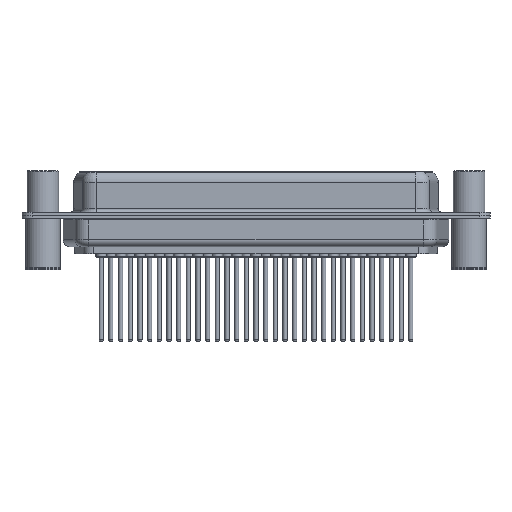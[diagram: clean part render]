
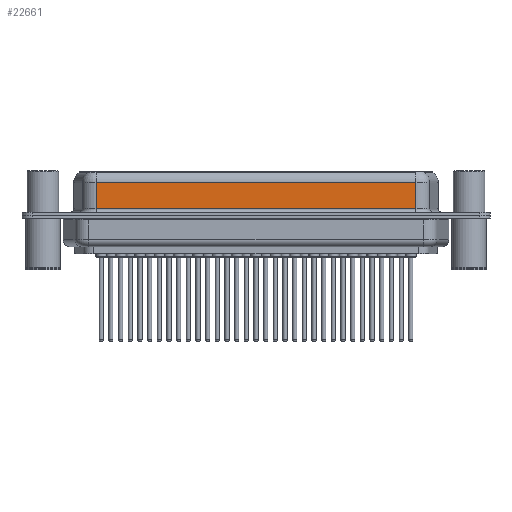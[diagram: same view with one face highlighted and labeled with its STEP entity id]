
A CAD part, front view. The second image highlights one B-rep face of the part: STEP entity #22661.
In plain terms, the highlighted planar face has unit normal (0, -1, 0).
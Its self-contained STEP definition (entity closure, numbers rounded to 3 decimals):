
#1103 = EDGE_CURVE ( 'NONE', #14342, #23252, #28003, .T. ) ;
#1141 = DIRECTION ( 'NONE',  ( 0., 0., -1. ) ) ;
#2949 = EDGE_CURVE ( 'NONE', #29314, #4065, #27001, .T. ) ;
#4065 = VERTEX_POINT ( 'NONE', #7651 ) ;
#4197 = VECTOR ( 'NONE', #24538, 1000. ) ;
#5983 = CARTESIAN_POINT ( 'NONE',  ( 53.383, -5.45, 4.65 ) ) ;
#6524 = LINE ( 'NONE', #5983, #13009 ) ;
#6656 = CARTESIAN_POINT ( 'NONE',  ( 7.617, -5.45, 6.4 ) ) ;
#6682 = DIRECTION ( 'NONE',  ( 0., 0., 1. ) ) ;
#7438 = CARTESIAN_POINT ( 'NONE',  ( 7.617, -5.45, 4.65 ) ) ;
#7651 = CARTESIAN_POINT ( 'NONE',  ( 53.383, -5.45, 0.9 ) ) ;
#9481 = CARTESIAN_POINT ( 'NONE',  ( 53.383, -5.45, 0.9 ) ) ;
#10989 = VECTOR ( 'NONE', #1141, 1000. ) ;
#11467 = DIRECTION ( 'NONE',  ( 0., 1., 0. ) ) ;
#11969 = VECTOR ( 'NONE', #25739, 1000. ) ;
#13009 = VECTOR ( 'NONE', #27520, 1000. ) ;
#14342 = VERTEX_POINT ( 'NONE', #7438 ) ;
#14460 = CARTESIAN_POINT ( 'NONE',  ( 53.383, -5.45, 6.4 ) ) ;
#15903 = CARTESIAN_POINT ( 'NONE',  ( 53.383, -5.45, 6.4 ) ) ;
#16544 = CARTESIAN_POINT ( 'NONE',  ( 7.617, -5.45, 0.9 ) ) ;
#17420 = ORIENTED_EDGE ( 'NONE', *, *, #32457, .T. ) ;
#19217 = PLANE ( 'NONE',  #21610 ) ;
#21610 = AXIS2_PLACEMENT_3D ( 'NONE', #14460, #11467, #6682 ) ;
#22350 = CARTESIAN_POINT ( 'NONE',  ( 53.383, -5.45, 4.65 ) ) ;
#22661 = ADVANCED_FACE ( 'NONE', ( #32604 ), #19217, .F. ) ;
#23252 = VERTEX_POINT ( 'NONE', #16544 ) ;
#24538 = DIRECTION ( 'NONE',  ( 0., 0., -1. ) ) ;
#25739 = DIRECTION ( 'NONE',  ( 1., 0., 0. ) ) ;
#27001 = LINE ( 'NONE', #15903, #4197 ) ;
#27520 = DIRECTION ( 'NONE',  ( -1., 0., 0. ) ) ;
#28003 = LINE ( 'NONE', #6656, #10989 ) ;
#28039 = ORIENTED_EDGE ( 'NONE', *, *, #28622, .T. ) ;
#28622 = EDGE_CURVE ( 'NONE', #29314, #14342, #6524, .T. ) ;
#29314 = VERTEX_POINT ( 'NONE', #22350 ) ;
#30159 = EDGE_LOOP ( 'NONE', ( #34354, #28039, #31643, #17420 ) ) ;
#31643 = ORIENTED_EDGE ( 'NONE', *, *, #1103, .T. ) ;
#32457 = EDGE_CURVE ( 'NONE', #23252, #4065, #34157, .T. ) ;
#32604 = FACE_OUTER_BOUND ( 'NONE', #30159, .T. ) ;
#34157 = LINE ( 'NONE', #9481, #11969 ) ;
#34354 = ORIENTED_EDGE ( 'NONE', *, *, #2949, .F. ) ;
